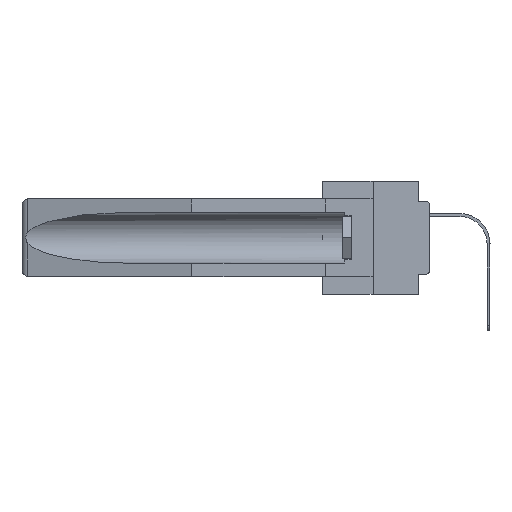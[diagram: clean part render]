
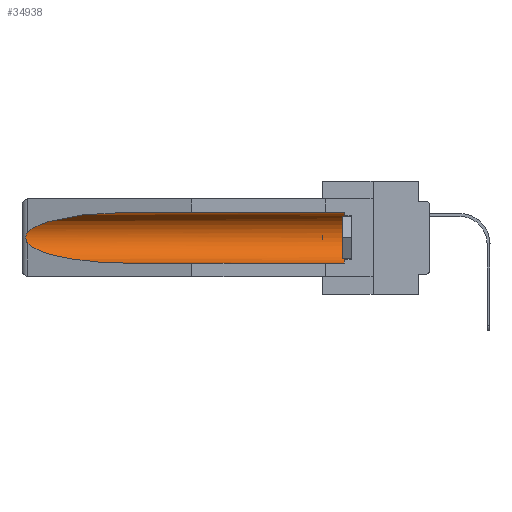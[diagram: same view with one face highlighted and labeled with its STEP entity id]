
A CAD part, left-side view. The second image highlights one B-rep face of the part: STEP entity #34938.
In plain terms, the highlighted cylindrical face has radius 2.857 mm (diameter 5.715 mm), a partial arc.
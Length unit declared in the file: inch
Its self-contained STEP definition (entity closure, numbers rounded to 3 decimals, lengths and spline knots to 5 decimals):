
#72 = EDGE_CURVE ( 'NONE', #20082, #26954, #20884, .T. ) ;
#543 = CARTESIAN_POINT ( 'NONE',  ( 0.26655, 1.53094, -0.18657 ) ) ;
#545 = EDGE_LOOP ( 'NONE', ( #21762, #6933, #25326, #27077, #10193, #30549 ) ) ;
#1643 = CARTESIAN_POINT ( 'NONE',  ( 0.26537, 1.52718, -0.14972 ) ) ;
#2182 = DIRECTION ( 'NONE',  ( 0., 1., 0. ) ) ;
#3349 = DIRECTION ( 'NONE',  ( 0., 0., 1. ) ) ;
#3541 = CARTESIAN_POINT ( 'NONE',  ( 0.2673, 1.5327, -0.16383 ) ) ;
#4228 = AXIS2_PLACEMENT_3D ( 'NONE', #25879, #28282, #35045 ) ;
#4268 = B_SPLINE_CURVE_WITH_KNOTS ( 'NONE', 3,
 ( #22205, #34351, #21621, #3541, #18822, #27974, #6721, #543, #6902, #25184 ),
 .UNSPECIFIED., .F., .F.,
 ( 4, 2, 2, 2, 4 ),
 ( 0., 0.00029, 0.00058, 0.00087, 0.00117 ),
 .UNSPECIFIED. ) ;
#4761 = CARTESIAN_POINT ( 'NONE',  ( 0.26537, 1.52718, -0.19328 ) ) ;
#5882 = CARTESIAN_POINT ( 'NONE',  ( 0.155, 0.126, -0.059 ) ) ;
#6015 = CARTESIAN_POINT ( 'NONE',  ( 0.26537, 1.52718, -0.19328 ) ) ;
#6721 = CARTESIAN_POINT ( 'NONE',  ( 0.2673, 1.53269, -0.17917 ) ) ;
#6902 = CARTESIAN_POINT ( 'NONE',  ( 0.26597, 1.5296, -0.19026 ) ) ;
#6933 = ORIENTED_EDGE ( 'NONE', *, *, #25030, .T. ) ;
#9813 = EDGE_CURVE ( 'NONE', #10971, #24317, #39239, .T. ) ;
#10193 = ORIENTED_EDGE ( 'NONE', *, *, #19450, .T. ) ;
#10971 = VERTEX_POINT ( 'NONE', #5882 ) ;
#11303 = CARTESIAN_POINT ( 'NONE',  ( 0.21114, 1.30732, -0.284 ) ) ;
#11346 = EDGE_CURVE ( 'NONE', #27907, #26954, #13411, .T. ) ;
#12415 = CARTESIAN_POINT ( 'NONE',  ( 0.155, -0.30754, -0.059 ) ) ;
#12571 = EDGE_CURVE ( 'NONE', #24317, #38569, #35410, .T. ) ;
#13411 = LINE ( 'NONE', #17296, #35168 ) ;
#15307 = CARTESIAN_POINT ( 'NONE',  ( 0.155, 0.126, -0.284 ) ) ;
#16172 = CYLINDRICAL_SURFACE ( 'NONE', #4228, 0.1125 ) ;
#16361 = FACE_OUTER_BOUND ( 'NONE', #545, .T. ) ;
#17062 = CARTESIAN_POINT ( 'NONE',  ( 0.25451, 1.48313, -0.24835 ) ) ;
#17296 = CARTESIAN_POINT ( 'NONE',  ( 0.155, -0.30754, -0.284 ) ) ;
#18565 = AXIS2_PLACEMENT_3D ( 'NONE', #33772, #24417, #3349 ) ;
#18822 = CARTESIAN_POINT ( 'NONE',  ( 0.2675, 1.53308, -0.16763 ) ) ;
#19450 = EDGE_CURVE ( 'NONE', #27907, #10971, #21758, .T. ) ;
#20082 = VERTEX_POINT ( 'NONE', #6015 ) ;
#20884 =( BOUNDED_CURVE ( )  B_SPLINE_CURVE ( 3, ( #4761, #17062, #11303, #28799 ),
 .UNSPECIFIED., .F., .T. ) 
 B_SPLINE_CURVE_WITH_KNOTS ( ( 4, 4 ),
 ( 0.1948, 1.5708 ),
 .UNSPECIFIED. ) 
 CURVE ( )  GEOMETRIC_REPRESENTATION_ITEM ( )  RATIONAL_B_SPLINE_CURVE ( ( 1., 0.848, 0.848, 1. ) ) 
 REPRESENTATION_ITEM ( '' )  );
#21621 = CARTESIAN_POINT ( 'NONE',  ( 0.26654, 1.53092, -0.15636 ) ) ;
#21758 = CIRCLE ( 'NONE', #18565, 0.1125 ) ;
#21762 = ORIENTED_EDGE ( 'NONE', *, *, #12571, .T. ) ;
#22205 = CARTESIAN_POINT ( 'NONE',  ( 0.26537, 1.52718, -0.14972 ) ) ;
#22933 = CARTESIAN_POINT ( 'NONE',  ( 0.155, 1.07973, -0.059 ) ) ;
#23130 = CARTESIAN_POINT ( 'NONE',  ( 0.21114, 1.30732, -0.059 ) ) ;
#24317 = VERTEX_POINT ( 'NONE', #32418 ) ;
#24417 = DIRECTION ( 'NONE',  ( 0., -1., 0. ) ) ;
#25030 = EDGE_CURVE ( 'NONE', #38569, #20082, #4268, .T. ) ;
#25184 = CARTESIAN_POINT ( 'NONE',  ( 0.26537, 1.52718, -0.19328 ) ) ;
#25326 = ORIENTED_EDGE ( 'NONE', *, *, #72, .T. ) ;
#25879 = CARTESIAN_POINT ( 'NONE',  ( 0.155, -0.30754, -0.1715 ) ) ;
#25903 = CARTESIAN_POINT ( 'NONE',  ( 0.25451, 1.48313, -0.09465 ) ) ;
#26954 = VERTEX_POINT ( 'NONE', #29743 ) ;
#27077 = ORIENTED_EDGE ( 'NONE', *, *, #11346, .F. ) ;
#27885 = DIRECTION ( 'NONE',  ( 0., 1., 0. ) ) ;
#27907 = VERTEX_POINT ( 'NONE', #15307 ) ;
#27974 = CARTESIAN_POINT ( 'NONE',  ( 0.2675, 1.53308, -0.17534 ) ) ;
#28282 = DIRECTION ( 'NONE',  ( 0., 1., 0. ) ) ;
#28799 = CARTESIAN_POINT ( 'NONE',  ( 0.155, 1.07973, -0.284 ) ) ;
#29743 = CARTESIAN_POINT ( 'NONE',  ( 0.155, 1.07973, -0.284 ) ) ;
#30549 = ORIENTED_EDGE ( 'NONE', *, *, #9813, .T. ) ;
#31784 = VECTOR ( 'NONE', #27885, 39.37008 ) ;
#32418 = CARTESIAN_POINT ( 'NONE',  ( 0.155, 1.07973, -0.059 ) ) ;
#33772 = CARTESIAN_POINT ( 'NONE',  ( 0.155, 0.126, -0.1715 ) ) ;
#34351 = CARTESIAN_POINT ( 'NONE',  ( 0.26597, 1.52961, -0.15275 ) ) ;
#34681 = CARTESIAN_POINT ( 'NONE',  ( 0.26537, 1.52718, -0.14972 ) ) ;
#34938 = ADVANCED_FACE ( 'NONE', ( #16361 ), #16172, .F. ) ;
#35045 = DIRECTION ( 'NONE',  ( 0., 0., 1. ) ) ;
#35168 = VECTOR ( 'NONE', #2182, 39.37008 ) ;
#35410 =( BOUNDED_CURVE ( )  B_SPLINE_CURVE ( 3, ( #22933, #23130, #25903, #34681 ),
 .UNSPECIFIED., .F., .F. ) 
 B_SPLINE_CURVE_WITH_KNOTS ( ( 4, 4 ),
 ( 4.71239, 6.08839 ),
 .UNSPECIFIED. ) 
 CURVE ( )  GEOMETRIC_REPRESENTATION_ITEM ( )  RATIONAL_B_SPLINE_CURVE ( ( 1., 0.848, 0.848, 1. ) ) 
 REPRESENTATION_ITEM ( '' )  );
#38569 = VERTEX_POINT ( 'NONE', #1643 ) ;
#39239 = LINE ( 'NONE', #12415, #31784 ) ;
